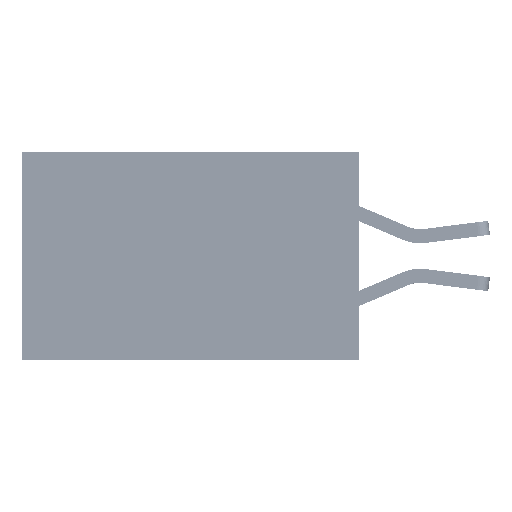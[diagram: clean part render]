
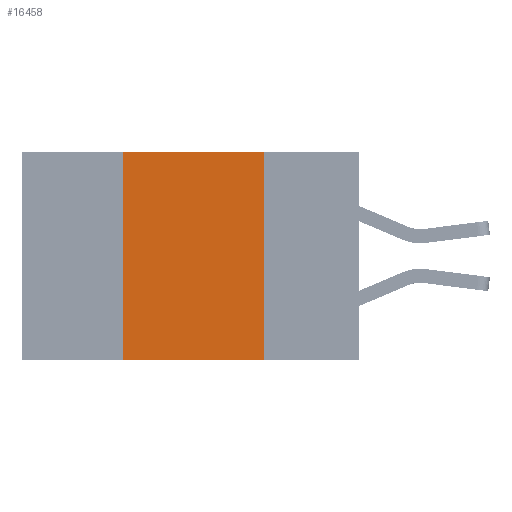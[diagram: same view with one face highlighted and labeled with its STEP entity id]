
A CAD part, left-side view. The second image highlights one B-rep face of the part: STEP entity #16458.
In plain terms, the highlighted planar face has unit normal (-1, 0, 0).
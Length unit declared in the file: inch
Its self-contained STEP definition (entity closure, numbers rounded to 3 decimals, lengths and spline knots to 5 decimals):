
#409 = VECTOR ( 'NONE', #9706, 39.37008 ) ;
#2290 = LINE ( 'NONE', #9825, #409 ) ;
#4057 = PLANE ( 'NONE',  #15378 ) ;
#4244 = DIRECTION ( 'NONE',  ( 0., -1., 0. ) ) ;
#4903 = CARTESIAN_POINT ( 'NONE',  ( 0., 0.42, -0.37 ) ) ;
#5631 = EDGE_CURVE ( 'NONE', #20370, #10590, #16756, .T. ) ;
#6171 = CARTESIAN_POINT ( 'NONE',  ( 0., 0.17, 0. ) ) ;
#7359 = CARTESIAN_POINT ( 'NONE',  ( 0., 0.6, 0. ) ) ;
#7930 = EDGE_LOOP ( 'NONE', ( #31529, #34840, #27609, #9646 ) ) ;
#8441 = EDGE_CURVE ( 'NONE', #8953, #17865, #18300, .T. ) ;
#8692 = VECTOR ( 'NONE', #4244, 39.37008 ) ;
#8953 = VERTEX_POINT ( 'NONE', #4903 ) ;
#9646 = ORIENTED_EDGE ( 'NONE', *, *, #10007, .T. ) ;
#9706 = DIRECTION ( 'NONE',  ( 0., -1., 0. ) ) ;
#9816 = DIRECTION ( 'NONE',  ( 0., 0., -1. ) ) ;
#9825 = CARTESIAN_POINT ( 'NONE',  ( 0., 0.6, 0. ) ) ;
#10007 = EDGE_CURVE ( 'NONE', #8953, #10590, #30373, .T. ) ;
#10465 = CARTESIAN_POINT ( 'NONE',  ( 0., 0.42, 0. ) ) ;
#10590 = VERTEX_POINT ( 'NONE', #36336 ) ;
#11360 = EDGE_CURVE ( 'NONE', #17865, #20370, #2290, .T. ) ;
#14090 = VECTOR ( 'NONE', #9816, 39.37008 ) ;
#15118 = VECTOR ( 'NONE', #30717, 39.37008 ) ;
#15378 = AXIS2_PLACEMENT_3D ( 'NONE', #7359, #20320, #15745 ) ;
#15745 = DIRECTION ( 'NONE',  ( 0., 0., -1. ) ) ;
#16458 = ADVANCED_FACE ( 'NONE', ( #24650 ), #4057, .F. ) ;
#16756 = LINE ( 'NONE', #6171, #14090 ) ;
#17865 = VERTEX_POINT ( 'NONE', #24904 ) ;
#18300 = LINE ( 'NONE', #10465, #15118 ) ;
#20320 = DIRECTION ( 'NONE',  ( 1., 0., 0. ) ) ;
#20370 = VERTEX_POINT ( 'NONE', #22227 ) ;
#22227 = CARTESIAN_POINT ( 'NONE',  ( 0., 0.17, 0. ) ) ;
#24650 = FACE_OUTER_BOUND ( 'NONE', #7930, .T. ) ;
#24904 = CARTESIAN_POINT ( 'NONE',  ( 0., 0.42, 0. ) ) ;
#27609 = ORIENTED_EDGE ( 'NONE', *, *, #8441, .F. ) ;
#30373 = LINE ( 'NONE', #36243, #8692 ) ;
#30717 = DIRECTION ( 'NONE',  ( 0., 0., 1. ) ) ;
#31529 = ORIENTED_EDGE ( 'NONE', *, *, #5631, .F. ) ;
#34840 = ORIENTED_EDGE ( 'NONE', *, *, #11360, .F. ) ;
#36243 = CARTESIAN_POINT ( 'NONE',  ( 0., 0.6, -0.37 ) ) ;
#36336 = CARTESIAN_POINT ( 'NONE',  ( 0., 0.17, -0.37 ) ) ;
